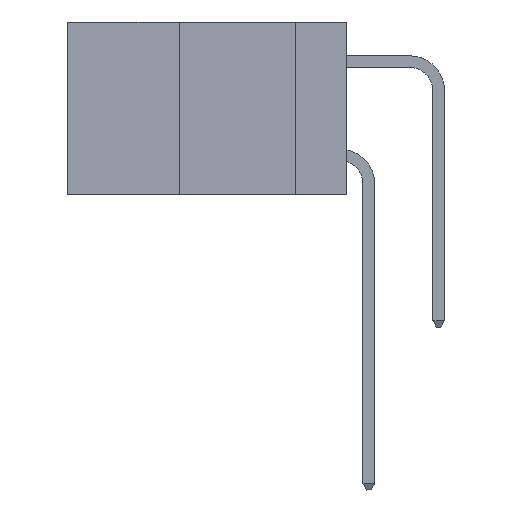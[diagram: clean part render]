
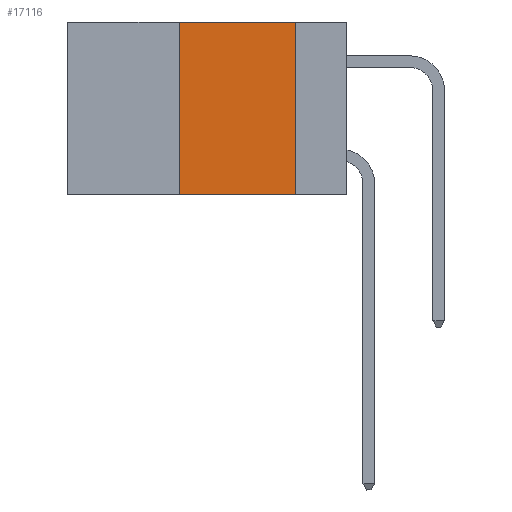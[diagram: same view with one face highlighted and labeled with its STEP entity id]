
A CAD part, left-side view. The second image highlights one B-rep face of the part: STEP entity #17116.
In plain terms, the highlighted planar face has unit normal (-1, 0, 0).
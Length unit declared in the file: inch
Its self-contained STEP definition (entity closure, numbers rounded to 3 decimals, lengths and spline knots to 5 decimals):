
#57 = EDGE_CURVE ( 'NONE', #20510, #14970, #4440, .T. ) ;
#1706 = CARTESIAN_POINT ( 'NONE',  ( 0., 0.6, 0. ) ) ;
#2447 = VERTEX_POINT ( 'NONE', #5707 ) ;
#3678 = DIRECTION ( 'NONE',  ( 0., 0., -1. ) ) ;
#4440 = LINE ( 'NONE', #6062, #9492 ) ;
#5707 = CARTESIAN_POINT ( 'NONE',  ( 0., 0.11, -0.37 ) ) ;
#6062 = CARTESIAN_POINT ( 'NONE',  ( 0., 0.36, 0. ) ) ;
#6582 = CARTESIAN_POINT ( 'NONE',  ( 0., 0.11, 0. ) ) ;
#7047 = EDGE_CURVE ( 'NONE', #20510, #2447, #19227, .T. ) ;
#7257 = CARTESIAN_POINT ( 'NONE',  ( 0., 0.36, 0. ) ) ;
#9345 = CARTESIAN_POINT ( 'NONE',  ( 0., 0.6, 0. ) ) ;
#9443 = ORIENTED_EDGE ( 'NONE', *, *, #15593, .F. ) ;
#9492 = VECTOR ( 'NONE', #19481, 39.37008 ) ;
#9568 = CARTESIAN_POINT ( 'NONE',  ( 0., 0.11, 0. ) ) ;
#9833 = ORIENTED_EDGE ( 'NONE', *, *, #20445, .F. ) ;
#9897 = VECTOR ( 'NONE', #23777, 39.37008 ) ;
#10145 = ORIENTED_EDGE ( 'NONE', *, *, #7047, .T. ) ;
#10213 = DIRECTION ( 'NONE',  ( 0., -1., 0. ) ) ;
#10383 = VECTOR ( 'NONE', #11281, 39.37008 ) ;
#10500 = ORIENTED_EDGE ( 'NONE', *, *, #57, .F. ) ;
#10516 = LINE ( 'NONE', #6582, #9897 ) ;
#11281 = DIRECTION ( 'NONE',  ( 0., -1., 0. ) ) ;
#11285 = PLANE ( 'NONE',  #19486 ) ;
#13228 = VERTEX_POINT ( 'NONE', #9568 ) ;
#14970 = VERTEX_POINT ( 'NONE', #7257 ) ;
#15178 = DIRECTION ( 'NONE',  ( 1., 0., 0. ) ) ;
#15593 = EDGE_CURVE ( 'NONE', #13228, #2447, #10516, .T. ) ;
#16123 = LINE ( 'NONE', #9345, #10383 ) ;
#17116 = ADVANCED_FACE ( 'NONE', ( #24822 ), #11285, .F. ) ;
#19227 = LINE ( 'NONE', #23669, #24317 ) ;
#19481 = DIRECTION ( 'NONE',  ( 0., 0., 1. ) ) ;
#19486 = AXIS2_PLACEMENT_3D ( 'NONE', #1706, #15178, #3678 ) ;
#20445 = EDGE_CURVE ( 'NONE', #14970, #13228, #16123, .T. ) ;
#20510 = VERTEX_POINT ( 'NONE', #21040 ) ;
#21040 = CARTESIAN_POINT ( 'NONE',  ( 0., 0.36, -0.37 ) ) ;
#23669 = CARTESIAN_POINT ( 'NONE',  ( 0., 0.6, -0.37 ) ) ;
#23777 = DIRECTION ( 'NONE',  ( 0., 0., -1. ) ) ;
#24317 = VECTOR ( 'NONE', #10213, 39.37008 ) ;
#24746 = EDGE_LOOP ( 'NONE', ( #9443, #9833, #10500, #10145 ) ) ;
#24822 = FACE_OUTER_BOUND ( 'NONE', #24746, .T. ) ;
